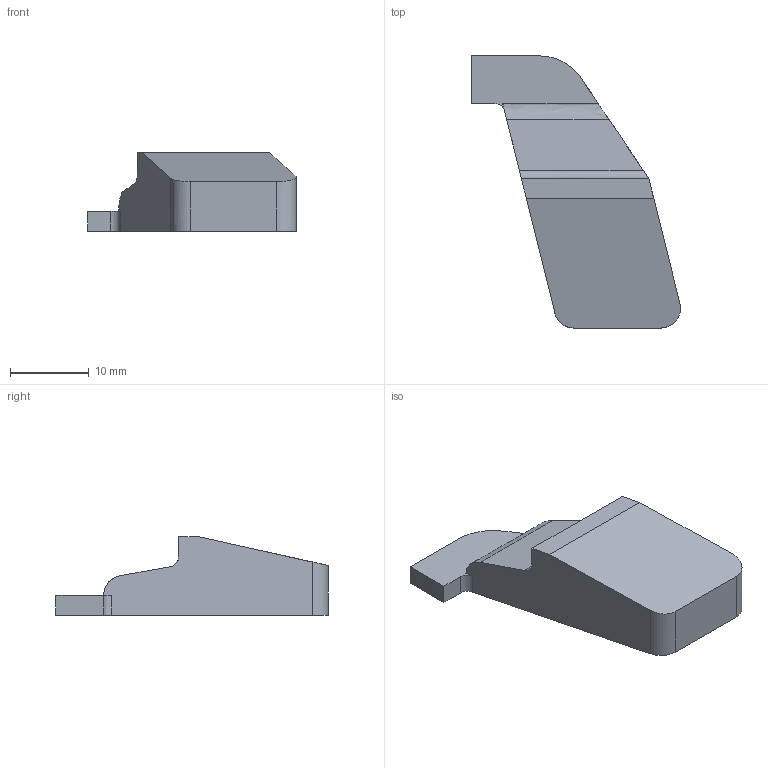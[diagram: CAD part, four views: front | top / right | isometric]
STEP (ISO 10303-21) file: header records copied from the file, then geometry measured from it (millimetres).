
FILE_DESCRIPTION (( 'STEP AP203' ), '1' );
FILE_NAME ('AR-9 Ejector V1.0.STEP', '2021-12-24T01:32:02', ( '' ), ( '' ), 'SwSTEP 2.0', 'SolidWorks 2021', '' );
FILE_SCHEMA (( 'CONFIG_CONTROL_DESIGN' ));
Length unit declared in the file: inch
Products named in the file (1): AR-9 Ejector V1.0
Bounding box: 26.62 x 34.67 x 10.03 mm (x, y, z)
Volume: 3548.3 mm3; surface area: 1742.7 mm2
Topology: 1 solids, 1 shells, 62 faces, 164 edges, 109 vertices
Faces by surface type: bspline 32, plane 24, cylinder 6
Entity records: 3391 total; most frequent: CARTESIAN_POINT 1998, ORIENTED_EDGE 328, DIRECTION 166, EDGE_CURVE 164, VERTEX_POINT 109, LINE 88, VECTOR 88, EDGE_LOOP 67
